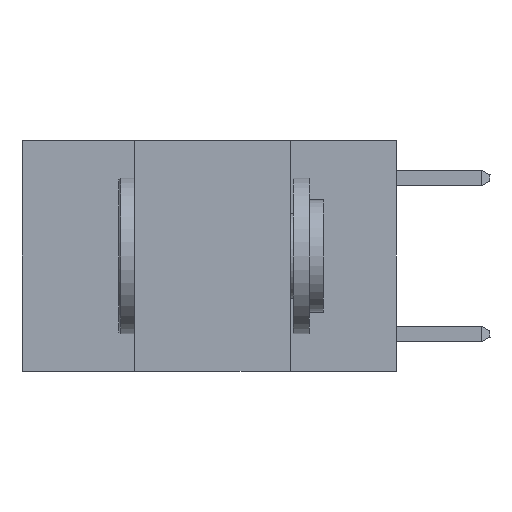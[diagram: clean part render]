
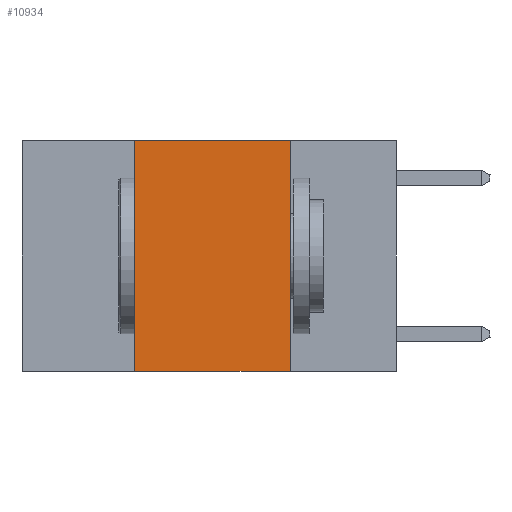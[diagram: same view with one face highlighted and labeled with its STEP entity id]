
A CAD part, left-side view. The second image highlights one B-rep face of the part: STEP entity #10934.
In plain terms, the highlighted planar face has unit normal (-1, 0, 0).
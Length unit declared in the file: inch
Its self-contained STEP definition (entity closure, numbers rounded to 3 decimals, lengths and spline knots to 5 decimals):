
#16 = EDGE_LOOP ( 'NONE', ( #3856, #8796, #11984, #7945 ) ) ;
#167 = VECTOR ( 'NONE', #5672, 39.37008 ) ;
#401 = LINE ( 'NONE', #6876, #9534 ) ;
#692 = VERTEX_POINT ( 'NONE', #5611 ) ;
#756 = CARTESIAN_POINT ( 'NONE',  ( 0., 0.42, 0. ) ) ;
#954 = CARTESIAN_POINT ( 'NONE',  ( 0., 0.6, 0. ) ) ;
#1587 = DIRECTION ( 'NONE',  ( 1., 0., 0. ) ) ;
#1653 = PLANE ( 'NONE',  #7458 ) ;
#2764 = VECTOR ( 'NONE', #8357, 39.37008 ) ;
#2836 = DIRECTION ( 'NONE',  ( 0., 0., 1. ) ) ;
#3049 = EDGE_CURVE ( 'NONE', #4611, #692, #401, .T. ) ;
#3272 = CARTESIAN_POINT ( 'NONE',  ( 0., 0.17, 0. ) ) ;
#3856 = ORIENTED_EDGE ( 'NONE', *, *, #11094, .F. ) ;
#4588 = CARTESIAN_POINT ( 'NONE',  ( 0., 0.17, 0. ) ) ;
#4611 = VERTEX_POINT ( 'NONE', #7963 ) ;
#5611 = CARTESIAN_POINT ( 'NONE',  ( 0., 0.17, -0.37 ) ) ;
#5621 = LINE ( 'NONE', #954, #167 ) ;
#5637 = LINE ( 'NONE', #4588, #2764 ) ;
#5672 = DIRECTION ( 'NONE',  ( 0., -1., 0. ) ) ;
#6876 = CARTESIAN_POINT ( 'NONE',  ( 0., 0.6, -0.37 ) ) ;
#7247 = CARTESIAN_POINT ( 'NONE',  ( 0., 0.6, 0. ) ) ;
#7458 = AXIS2_PLACEMENT_3D ( 'NONE', #7247, #1587, #7989 ) ;
#7484 = VECTOR ( 'NONE', #2836, 39.37008 ) ;
#7538 = CARTESIAN_POINT ( 'NONE',  ( 0., 0.42, 0. ) ) ;
#7945 = ORIENTED_EDGE ( 'NONE', *, *, #3049, .T. ) ;
#7963 = CARTESIAN_POINT ( 'NONE',  ( 0., 0.42, -0.37 ) ) ;
#7989 = DIRECTION ( 'NONE',  ( 0., 0., -1. ) ) ;
#8055 = FACE_OUTER_BOUND ( 'NONE', #16, .T. ) ;
#8357 = DIRECTION ( 'NONE',  ( 0., 0., -1. ) ) ;
#8468 = EDGE_CURVE ( 'NONE', #8727, #11774, #5621, .T. ) ;
#8645 = DIRECTION ( 'NONE',  ( 0., -1., 0. ) ) ;
#8727 = VERTEX_POINT ( 'NONE', #756 ) ;
#8796 = ORIENTED_EDGE ( 'NONE', *, *, #8468, .F. ) ;
#9501 = LINE ( 'NONE', #7538, #7484 ) ;
#9534 = VECTOR ( 'NONE', #8645, 39.37008 ) ;
#10934 = ADVANCED_FACE ( 'NONE', ( #8055 ), #1653, .F. ) ;
#11094 = EDGE_CURVE ( 'NONE', #11774, #692, #5637, .T. ) ;
#11774 = VERTEX_POINT ( 'NONE', #3272 ) ;
#11984 = ORIENTED_EDGE ( 'NONE', *, *, #12071, .F. ) ;
#12071 = EDGE_CURVE ( 'NONE', #4611, #8727, #9501, .T. ) ;
